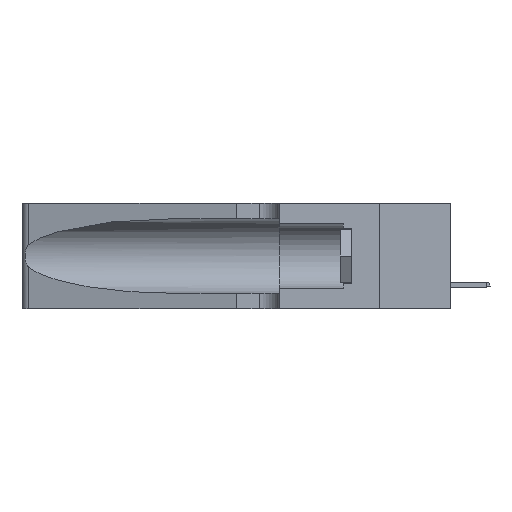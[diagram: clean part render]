
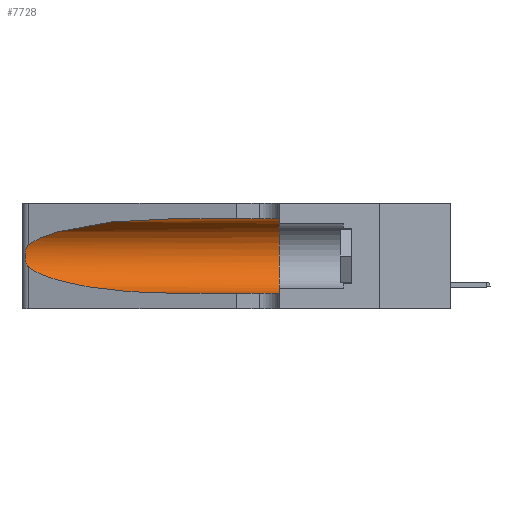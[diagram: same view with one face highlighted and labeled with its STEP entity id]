
A CAD part, left-side view. The second image highlights one B-rep face of the part: STEP entity #7728.
In plain terms, the highlighted cylindrical face has radius 3.308 mm (diameter 6.617 mm), a partial arc.
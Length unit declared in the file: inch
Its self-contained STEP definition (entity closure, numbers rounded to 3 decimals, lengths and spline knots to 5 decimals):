
#289 = EDGE_CURVE ( 'NONE', #3173, #17940, #13792, .T. ) ;
#447 = CARTESIAN_POINT ( 'NONE',  ( 0.1305, 1.61858, 0.185 ) ) ;
#539 = DIRECTION ( 'NONE',  ( 0., 1., 0. ) ) ;
#778 = CARTESIAN_POINT ( 'NONE',  ( 0.26018, 1.23835, 0.19895 ) ) ;
#835 = ORIENTED_EDGE ( 'NONE', *, *, #17602, .T. ) ;
#1088 = CARTESIAN_POINT ( 'NONE',  ( 0.25639, 1.23186, 0.15144 ) ) ;
#1593 = ORIENTED_EDGE ( 'NONE', *, *, #18213, .F. ) ;
#1848 = ORIENTED_EDGE ( 'NONE', *, *, #15445, .T. ) ;
#1870 = DIRECTION ( 'NONE',  ( 0., -1., 0. ) ) ;
#1899 = DIRECTION ( 'NONE',  ( 0., 0., 1. ) ) ;
#2078 = VERTEX_POINT ( 'NONE', #4192 ) ;
#2342 = CARTESIAN_POINT ( 'NONE',  ( 0.25555, 1.22994, 0.2215 ) ) ;
#2463 = EDGE_CURVE ( 'NONE', #17940, #5079, #13580, .T. ) ;
#3032 = CARTESIAN_POINT ( 'NONE',  ( 0.2373, 1.15595, 0.28018 ) ) ;
#3173 = VERTEX_POINT ( 'NONE', #19302 ) ;
#3535 = LINE ( 'NONE', #17854, #9495 ) ;
#3854 = CARTESIAN_POINT ( 'NONE',  ( 0.1305, 0.35, 0.31525 ) ) ;
#3999 = CARTESIAN_POINT ( 'NONE',  ( 0.25856, 1.23593, 0.16098 ) ) ;
#4192 = CARTESIAN_POINT ( 'NONE',  ( 0.1305, 0.35, 0.05475 ) ) ;
#4298 = CARTESIAN_POINT ( 'NONE',  ( 0.18966, 0.96281, 0.31525 ) ) ;
#4580 = CARTESIAN_POINT ( 'NONE',  ( 0.1305, 1.61858, 0.05475 ) ) ;
#4581 = EDGE_LOOP ( 'NONE', ( #17542, #10667, #835, #1848, #7518, #1593 ) ) ;
#4709 = CARTESIAN_POINT ( 'NONE',  ( 0.2373, 1.15595, 0.08982 ) ) ;
#5079 = VERTEX_POINT ( 'NONE', #18907 ) ;
#5304 = VECTOR ( 'NONE', #6300, 39.37008 ) ;
#5376 = CARTESIAN_POINT ( 'NONE',  ( 0.25639, 1.23184, 0.21858 ) ) ;
#5377 = CIRCLE ( 'NONE', #8158, 0.13025 ) ;
#5588 = CARTESIAN_POINT ( 'NONE',  ( 0.26075, 1.23896, 0.178 ) ) ;
#6300 = DIRECTION ( 'NONE',  ( 0., -1., 0. ) ) ;
#6327 = CARTESIAN_POINT ( 'NONE',  ( 0.25487, 1.22718, 0.14631 ) ) ;
#7072 = DIRECTION ( 'NONE',  ( 0., -1., 0. ) ) ;
#7215 = CARTESIAN_POINT ( 'NONE',  ( 0.26075, 1.23896, 0.19203 ) ) ;
#7518 = ORIENTED_EDGE ( 'NONE', *, *, #19149, .F. ) ;
#7728 = ADVANCED_FACE ( 'NONE', ( #15122 ), #8295, .F. ) ;
#7966 = CARTESIAN_POINT ( 'NONE',  ( 0.25487, 1.22718, 0.22369 ) ) ;
#8158 = AXIS2_PLACEMENT_3D ( 'NONE', #16414, #539, #1899 ) ;
#8295 = CYLINDRICAL_SURFACE ( 'NONE', #18666, 0.13025 ) ;
#8811 = CARTESIAN_POINT ( 'NONE',  ( 0.25787, 1.23484, 0.2124 ) ) ;
#9097 = CARTESIAN_POINT ( 'NONE',  ( 0.1305, 0.72297, 0.31525 ) ) ;
#9495 = VECTOR ( 'NONE', #1870, 39.37008 ) ;
#9850 = VERTEX_POINT ( 'NONE', #11692 ) ;
#10544 = CARTESIAN_POINT ( 'NONE',  ( 0.25789, 1.23486, 0.15765 ) ) ;
#10667 = ORIENTED_EDGE ( 'NONE', *, *, #2463, .T. ) ;
#11152 = CARTESIAN_POINT ( 'NONE',  ( 0.18966, 0.96281, 0.05475 ) ) ;
#11692 = CARTESIAN_POINT ( 'NONE',  ( 0.1305, 0.72297, 0.05475 ) ) ;
#12084 = CARTESIAN_POINT ( 'NONE',  ( 0.25487, 1.22718, 0.22369 ) ) ;
#12523 = CARTESIAN_POINT ( 'NONE',  ( 0.25555, 1.22993, 0.14849 ) ) ;
#13580 = B_SPLINE_CURVE_WITH_KNOTS ( 'NONE', 3,
 ( #16853, #2342, #5376, #8811, #15250, #778, #7215, #5588, #18522, #3999, #10544, #1088, #12523, #18954 ),
 .UNSPECIFIED., .F., .F.,
 ( 4, 2, 2, 2, 2, 2, 4 ),
 ( 0., 0.00027, 0.00053, 0.00107, 0.0016, 0.00187, 0.00214 ),
 .UNSPECIFIED. ) ;
#13792 =( BOUNDED_CURVE ( )  B_SPLINE_CURVE ( 3, ( #9097, #4298, #3032, #7966 ),
 .UNSPECIFIED., .F., .T. ) 
 B_SPLINE_CURVE_WITH_KNOTS ( ( 4, 4 ),
 ( 1.5708, 2.84003 ),
 .UNSPECIFIED. ) 
 CURVE ( )  GEOMETRIC_REPRESENTATION_ITEM ( )  RATIONAL_B_SPLINE_CURVE ( ( 1., 0.87, 0.87, 1. ) ) 
 REPRESENTATION_ITEM ( '' )  );
#14914 = DIRECTION ( 'NONE',  ( 0., 0., -1. ) ) ;
#15122 = FACE_OUTER_BOUND ( 'NONE', #4581, .T. ) ;
#15250 = CARTESIAN_POINT ( 'NONE',  ( 0.25854, 1.2359, 0.20912 ) ) ;
#15445 = EDGE_CURVE ( 'NONE', #9850, #2078, #15509, .T. ) ;
#15509 = LINE ( 'NONE', #4580, #5304 ) ;
#16414 = CARTESIAN_POINT ( 'NONE',  ( 0.1305, 0.35, 0.185 ) ) ;
#16497 = VERTEX_POINT ( 'NONE', #3854 ) ;
#16853 = CARTESIAN_POINT ( 'NONE',  ( 0.25487, 1.22718, 0.22369 ) ) ;
#17542 = ORIENTED_EDGE ( 'NONE', *, *, #289, .T. ) ;
#17602 = EDGE_CURVE ( 'NONE', #5079, #9850, #20251, .T. ) ;
#17675 = CARTESIAN_POINT ( 'NONE',  ( 0.1305, 0.72297, 0.05475 ) ) ;
#17854 = CARTESIAN_POINT ( 'NONE',  ( 0.1305, 1.61858, 0.31525 ) ) ;
#17940 = VERTEX_POINT ( 'NONE', #12084 ) ;
#18213 = EDGE_CURVE ( 'NONE', #3173, #16497, #3535, .T. ) ;
#18522 = CARTESIAN_POINT ( 'NONE',  ( 0.26017, 1.23833, 0.17102 ) ) ;
#18666 = AXIS2_PLACEMENT_3D ( 'NONE', #447, #7072, #14914 ) ;
#18907 = CARTESIAN_POINT ( 'NONE',  ( 0.25487, 1.22718, 0.14631 ) ) ;
#18954 = CARTESIAN_POINT ( 'NONE',  ( 0.25487, 1.22718, 0.14631 ) ) ;
#19149 = EDGE_CURVE ( 'NONE', #16497, #2078, #5377, .T. ) ;
#19302 = CARTESIAN_POINT ( 'NONE',  ( 0.1305, 0.72297, 0.31525 ) ) ;
#20251 =( BOUNDED_CURVE ( )  B_SPLINE_CURVE ( 3, ( #6327, #4709, #11152, #17675 ),
 .UNSPECIFIED., .F., .T. ) 
 B_SPLINE_CURVE_WITH_KNOTS ( ( 4, 4 ),
 ( 3.44316, 4.71239 ),
 .UNSPECIFIED. ) 
 CURVE ( )  GEOMETRIC_REPRESENTATION_ITEM ( )  RATIONAL_B_SPLINE_CURVE ( ( 1., 0.87, 0.87, 1. ) ) 
 REPRESENTATION_ITEM ( '' )  );
